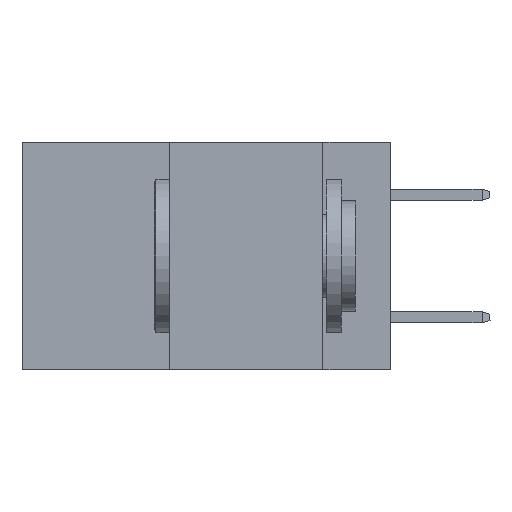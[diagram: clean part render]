
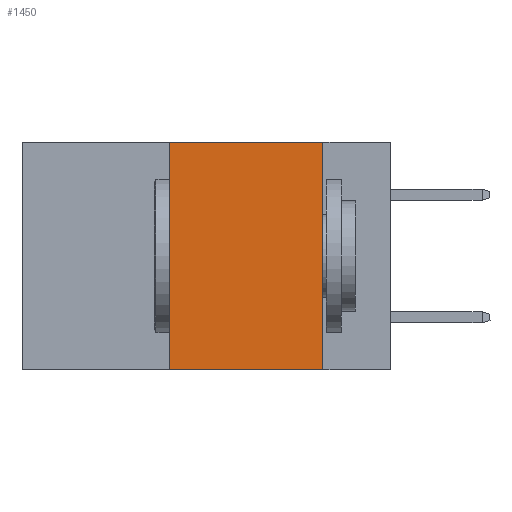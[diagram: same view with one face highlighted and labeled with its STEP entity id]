
A CAD part, left-side view. The second image highlights one B-rep face of the part: STEP entity #1450.
In plain terms, the highlighted planar face has unit normal (-1, 0, 0).
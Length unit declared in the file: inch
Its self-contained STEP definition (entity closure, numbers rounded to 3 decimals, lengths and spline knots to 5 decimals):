
#1225 = EDGE_CURVE ( 'NONE', #9206, #5796, #10465, .T. ) ;
#1358 = VECTOR ( 'NONE', #8235, 39.37008 ) ;
#1450 = ADVANCED_FACE ( 'NONE', ( #2136 ), #9116, .F. ) ;
#1491 = VECTOR ( 'NONE', #8672, 39.37008 ) ;
#1763 = DIRECTION ( 'NONE',  ( 0., 0., 1. ) ) ;
#1849 = CARTESIAN_POINT ( 'NONE',  ( 0., 0.11, 0. ) ) ;
#1875 = CARTESIAN_POINT ( 'NONE',  ( 0., 0.6, 0. ) ) ;
#1956 = LINE ( 'NONE', #4744, #3576 ) ;
#2040 = DIRECTION ( 'NONE',  ( 0., -1., 0. ) ) ;
#2136 = FACE_OUTER_BOUND ( 'NONE', #8143, .T. ) ;
#2727 = DIRECTION ( 'NONE',  ( 1., 0., 0. ) ) ;
#3313 = ORIENTED_EDGE ( 'NONE', *, *, #6661, .F. ) ;
#3384 = ORIENTED_EDGE ( 'NONE', *, *, #4558, .T. ) ;
#3449 = CARTESIAN_POINT ( 'NONE',  ( 0., 0.36, 0. ) ) ;
#3576 = VECTOR ( 'NONE', #2040, 39.37008 ) ;
#4558 = EDGE_CURVE ( 'NONE', #9621, #4779, #1956, .T. ) ;
#4718 = AXIS2_PLACEMENT_3D ( 'NONE', #6149, #2727, #10436 ) ;
#4744 = CARTESIAN_POINT ( 'NONE',  ( 0., 0.6, -0.37 ) ) ;
#4779 = VERTEX_POINT ( 'NONE', #5251 ) ;
#5251 = CARTESIAN_POINT ( 'NONE',  ( 0., 0.11, -0.37 ) ) ;
#5710 = CARTESIAN_POINT ( 'NONE',  ( 0., 0.11, 0. ) ) ;
#5796 = VERTEX_POINT ( 'NONE', #1849 ) ;
#6149 = CARTESIAN_POINT ( 'NONE',  ( 0., 0.6, 0. ) ) ;
#6305 = VECTOR ( 'NONE', #1763, 39.37008 ) ;
#6661 = EDGE_CURVE ( 'NONE', #5796, #4779, #6964, .T. ) ;
#6831 = CARTESIAN_POINT ( 'NONE',  ( 0., 0.36, 0. ) ) ;
#6903 = ORIENTED_EDGE ( 'NONE', *, *, #1225, .F. ) ;
#6964 = LINE ( 'NONE', #5710, #1358 ) ;
#7333 = EDGE_CURVE ( 'NONE', #9621, #9206, #8551, .T. ) ;
#8143 = EDGE_LOOP ( 'NONE', ( #3313, #6903, #8361, #3384 ) ) ;
#8235 = DIRECTION ( 'NONE',  ( 0., 0., -1. ) ) ;
#8361 = ORIENTED_EDGE ( 'NONE', *, *, #7333, .F. ) ;
#8551 = LINE ( 'NONE', #3449, #6305 ) ;
#8672 = DIRECTION ( 'NONE',  ( 0., -1., 0. ) ) ;
#9116 = PLANE ( 'NONE',  #4718 ) ;
#9206 = VERTEX_POINT ( 'NONE', #6831 ) ;
#9621 = VERTEX_POINT ( 'NONE', #9646 ) ;
#9646 = CARTESIAN_POINT ( 'NONE',  ( 0., 0.36, -0.37 ) ) ;
#10436 = DIRECTION ( 'NONE',  ( 0., 0., -1. ) ) ;
#10465 = LINE ( 'NONE', #1875, #1491 ) ;
